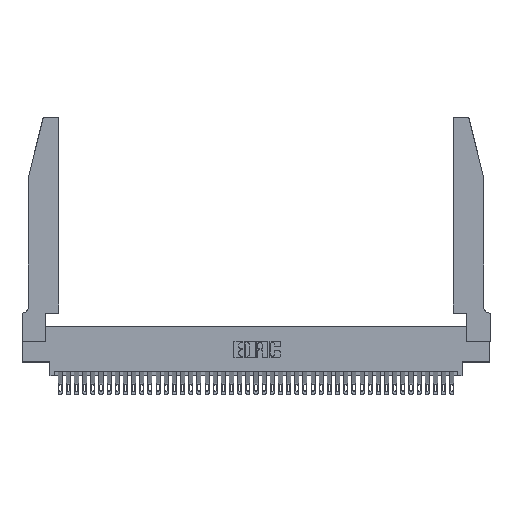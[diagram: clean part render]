
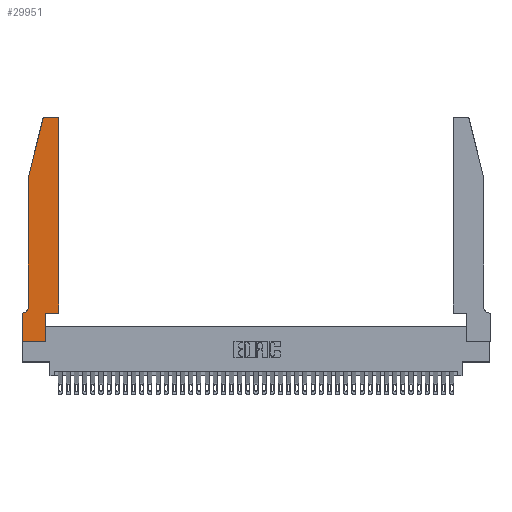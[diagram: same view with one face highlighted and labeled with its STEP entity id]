
A CAD part, top view. The second image highlights one B-rep face of the part: STEP entity #29951.
In plain terms, the highlighted planar face has unit normal (0, 0, 1).
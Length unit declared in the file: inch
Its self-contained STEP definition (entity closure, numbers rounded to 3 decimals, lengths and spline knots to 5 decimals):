
#150 = EDGE_CURVE ( 'NONE', #23093, #3857, #31747, .T. ) ;
#452 = DIRECTION ( 'NONE',  ( 0., 0., -1. ) ) ;
#537 = VERTEX_POINT ( 'NONE', #33639 ) ;
#786 = CARTESIAN_POINT ( 'NONE',  ( 0.0755, 2., 0.37 ) ) ;
#1649 = CARTESIAN_POINT ( 'NONE',  ( 0.2605, 2.75, 0.37 ) ) ;
#1795 = VERTEX_POINT ( 'NONE', #35378 ) ;
#2258 = DIRECTION ( 'NONE',  ( 0., 0., 1. ) ) ;
#2303 = PLANE ( 'NONE',  #34960 ) ;
#2663 = CARTESIAN_POINT ( 'NONE',  ( 0.25487, 2.72718, 0.37 ) ) ;
#3206 = EDGE_CURVE ( 'NONE', #6315, #19415, #26440, .T. ) ;
#3857 = VERTEX_POINT ( 'NONE', #38882 ) ;
#4655 = DIRECTION ( 'NONE',  ( -1., 0., 0. ) ) ;
#6230 = ORIENTED_EDGE ( 'NONE', *, *, #35084, .T. ) ;
#6315 = VERTEX_POINT ( 'NONE', #20222 ) ;
#7063 = CARTESIAN_POINT ( 'NONE',  ( 0.0755, 0.35, 0.37 ) ) ;
#7585 = DIRECTION ( 'NONE',  ( 0., 1., 0. ) ) ;
#8623 = EDGE_CURVE ( 'NONE', #33062, #9715, #23119, .T. ) ;
#9137 = ORIENTED_EDGE ( 'NONE', *, *, #14164, .T. ) ;
#9715 = VERTEX_POINT ( 'NONE', #29563 ) ;
#10242 = LINE ( 'NONE', #7063, #16929 ) ;
#10917 = DIRECTION ( 'NONE',  ( -0.239, -0.971, 0. ) ) ;
#11011 = VECTOR ( 'NONE', #7585, 39.37008 ) ;
#11659 = DIRECTION ( 'NONE',  ( 1., 0., 0. ) ) ;
#11782 = EDGE_CURVE ( 'NONE', #9715, #37213, #40706, .T. ) ;
#12227 = ORIENTED_EDGE ( 'NONE', *, *, #150, .T. ) ;
#12794 = CARTESIAN_POINT ( 'NONE',  ( 0., 0., 0.37 ) ) ;
#13569 = LINE ( 'NONE', #32699, #11011 ) ;
#13614 = CARTESIAN_POINT ( 'NONE',  ( 0.0055, 0.35, 0.37 ) ) ;
#13866 = EDGE_CURVE ( 'NONE', #37213, #1795, #36863, .T. ) ;
#14164 = EDGE_CURVE ( 'NONE', #19415, #18306, #13569, .T. ) ;
#14246 = CARTESIAN_POINT ( 'NONE',  ( 0.0755, 2., 0.37 ) ) ;
#14277 = VERTEX_POINT ( 'NONE', #32529 ) ;
#14332 = VECTOR ( 'NONE', #4655, 39.37008 ) ;
#15120 = CARTESIAN_POINT ( 'NONE',  ( 0.4505, 0.35, 0.37 ) ) ;
#15166 = CARTESIAN_POINT ( 'NONE',  ( 0.284, 2.72, 0.37 ) ) ;
#16896 = EDGE_LOOP ( 'NONE', ( #38481, #42243, #23411, #27317, #40107, #6230, #12227, #30087, #39374, #36678, #9137, #30532 ) ) ;
#16929 = VECTOR ( 'NONE', #17123, 39.37008 ) ;
#17123 = DIRECTION ( 'NONE',  ( -1., 0., 0. ) ) ;
#18253 = VECTOR ( 'NONE', #10917, 39.37008 ) ;
#18306 = VERTEX_POINT ( 'NONE', #28737 ) ;
#18385 = DIRECTION ( 'NONE',  ( 1., 0., 0. ) ) ;
#18519 = LINE ( 'NONE', #30886, #19596 ) ;
#18968 = CARTESIAN_POINT ( 'NONE',  ( 0., 0.35, 0.37 ) ) ;
#19415 = VERTEX_POINT ( 'NONE', #15120 ) ;
#19596 = VECTOR ( 'NONE', #31031, 39.37008 ) ;
#19875 = DIRECTION ( 'NONE',  ( 0., -1., 0. ) ) ;
#20222 = CARTESIAN_POINT ( 'NONE',  ( 0.2865, 0.35, 0.37 ) ) ;
#20259 = CARTESIAN_POINT ( 'NONE',  ( 0.0055, 0.42, 0.37 ) ) ;
#20745 = CARTESIAN_POINT ( 'NONE',  ( 0., 0.35, 0.37 ) ) ;
#20920 = DIRECTION ( 'NONE',  ( 0., -1., 0. ) ) ;
#21073 = LINE ( 'NONE', #38073, #23614 ) ;
#21892 = EDGE_CURVE ( 'NONE', #14277, #6315, #18519, .T. ) ;
#21920 = VECTOR ( 'NONE', #19875, 39.37008 ) ;
#22405 = VECTOR ( 'NONE', #20920, 39.37008 ) ;
#22613 = DIRECTION ( 'NONE',  ( 0., 0., 1. ) ) ;
#23093 = VERTEX_POINT ( 'NONE', #20745 ) ;
#23119 = LINE ( 'NONE', #1649, #14332 ) ;
#23411 = ORIENTED_EDGE ( 'NONE', *, *, #13866, .T. ) ;
#23559 = DIRECTION ( 'NONE',  ( -1., 0., 0. ) ) ;
#23614 = VECTOR ( 'NONE', #11659, 39.37008 ) ;
#23819 = CIRCLE ( 'NONE', #30736, 0.03 ) ;
#25339 = DIRECTION ( 'NONE',  ( 1., 0., 0. ) ) ;
#26440 = LINE ( 'NONE', #35929, #39798 ) ;
#27317 = ORIENTED_EDGE ( 'NONE', *, *, #37646, .T. ) ;
#28737 = CARTESIAN_POINT ( 'NONE',  ( 0.4505, 2.72, 0.37 ) ) ;
#29563 = CARTESIAN_POINT ( 'NONE',  ( 0.284, 2.75, 0.37 ) ) ;
#29951 = ADVANCED_FACE ( 'NONE', ( #33754 ), #2303, .T. ) ;
#30087 = ORIENTED_EDGE ( 'NONE', *, *, #35339, .T. ) ;
#30532 = ORIENTED_EDGE ( 'NONE', *, *, #33410, .T. ) ;
#30736 = AXIS2_PLACEMENT_3D ( 'NONE', #35761, #22613, #38827 ) ;
#30886 = CARTESIAN_POINT ( 'NONE',  ( 0.2865, 0.35, 0.37 ) ) ;
#31031 = DIRECTION ( 'NONE',  ( 0., 1., 0. ) ) ;
#31747 = LINE ( 'NONE', #12794, #21920 ) ;
#32007 = DIRECTION ( 'NONE',  ( 1., 0., 0. ) ) ;
#32039 = VERTEX_POINT ( 'NONE', #13614 ) ;
#32156 = DIRECTION ( 'NONE',  ( 0., 0., 1. ) ) ;
#32529 = CARTESIAN_POINT ( 'NONE',  ( 0.2865, 0., 0.37 ) ) ;
#32699 = CARTESIAN_POINT ( 'NONE',  ( 0.4505, 0.35, 0.37 ) ) ;
#33062 = VERTEX_POINT ( 'NONE', #33483 ) ;
#33410 = EDGE_CURVE ( 'NONE', #18306, #33062, #23819, .T. ) ;
#33483 = CARTESIAN_POINT ( 'NONE',  ( 0.4205, 2.75, 0.37 ) ) ;
#33639 = CARTESIAN_POINT ( 'NONE',  ( 0.0755, 0.42, 0.37 ) ) ;
#33754 = FACE_OUTER_BOUND ( 'NONE', #16896, .T. ) ;
#34370 = AXIS2_PLACEMENT_3D ( 'NONE', #20259, #452, #23559 ) ;
#34960 = AXIS2_PLACEMENT_3D ( 'NONE', #18968, #32156, #18385 ) ;
#35084 = EDGE_CURVE ( 'NONE', #32039, #23093, #10242, .T. ) ;
#35339 = EDGE_CURVE ( 'NONE', #3857, #14277, #21073, .T. ) ;
#35378 = CARTESIAN_POINT ( 'NONE',  ( 0.0755, 2., 0.37 ) ) ;
#35761 = CARTESIAN_POINT ( 'NONE',  ( 0.4205, 2.72, 0.37 ) ) ;
#35929 = CARTESIAN_POINT ( 'NONE',  ( 0.4505, 0.35, 0.37 ) ) ;
#36678 = ORIENTED_EDGE ( 'NONE', *, *, #3206, .T. ) ;
#36821 = EDGE_CURVE ( 'NONE', #537, #32039, #39568, .T. ) ;
#36863 = LINE ( 'NONE', #786, #18253 ) ;
#36874 = LINE ( 'NONE', #14246, #22405 ) ;
#37213 = VERTEX_POINT ( 'NONE', #2663 ) ;
#37646 = EDGE_CURVE ( 'NONE', #1795, #537, #36874, .T. ) ;
#38073 = CARTESIAN_POINT ( 'NONE',  ( 0., 0., 0.37 ) ) ;
#38481 = ORIENTED_EDGE ( 'NONE', *, *, #8623, .T. ) ;
#38827 = DIRECTION ( 'NONE',  ( 1., 0., 0. ) ) ;
#38882 = CARTESIAN_POINT ( 'NONE',  ( 0., 0., 0.37 ) ) ;
#39374 = ORIENTED_EDGE ( 'NONE', *, *, #21892, .T. ) ;
#39568 = CIRCLE ( 'NONE', #34370, 0.07 ) ;
#39798 = VECTOR ( 'NONE', #32007, 39.37008 ) ;
#40107 = ORIENTED_EDGE ( 'NONE', *, *, #36821, .T. ) ;
#40706 = CIRCLE ( 'NONE', #42508, 0.03 ) ;
#42243 = ORIENTED_EDGE ( 'NONE', *, *, #11782, .T. ) ;
#42508 = AXIS2_PLACEMENT_3D ( 'NONE', #15166, #2258, #25339 ) ;
